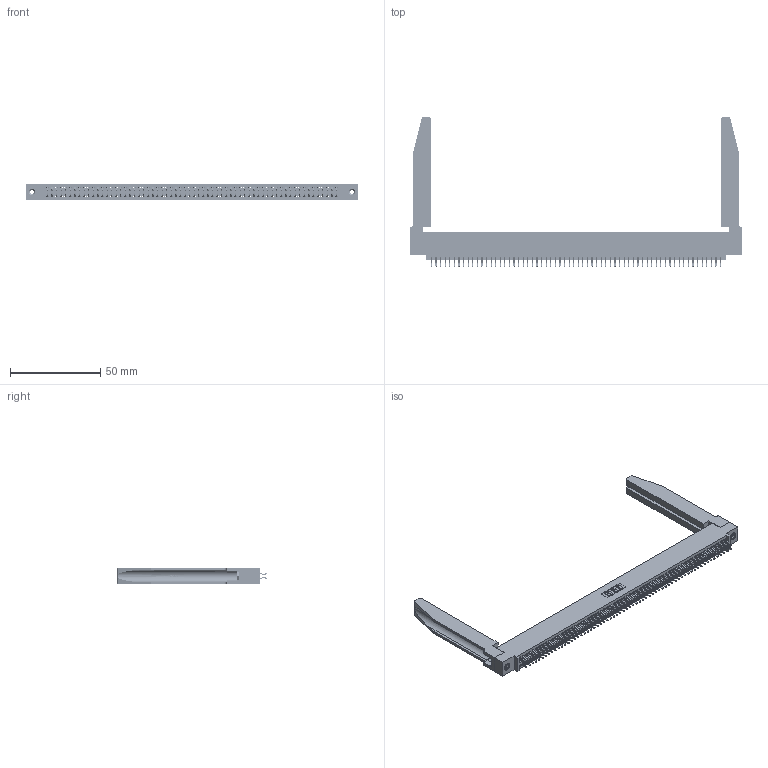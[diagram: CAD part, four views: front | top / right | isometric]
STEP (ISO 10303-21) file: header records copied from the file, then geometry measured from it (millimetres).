
FILE_DESCRIPTION (( 'STEP AP203' ), '1' );
FILE_NAME ('395-128-556-578.STEP', '2019-10-28T20:31:51', ( '' ), ( '' ), 'SwSTEP 2.0', 'SolidWorks 2016', '' );
FILE_SCHEMA (( 'CONFIG_CONTROL_DESIGN' ));
Length unit declared in the file: inch
Products named in the file (5): 345 Part_0.110 Offset - 0.156 Dia-TH; 345-292-001_556 Tail; 345-250-001_345-250-001-102; 345-220-078_345-220-078; 395-128-556-578
Assembly tree (133 placements, depth 2):
  395-128-556-578
    345 Part_0.110 Offset - 0.156 Dia-TH
    345-292-001_556 Tail  x128
    345-250-001_345-250-001-102  x2
    345-220-078_345-220-078  x2
Bounding box: 183.79 x 82.99 x 9.4 mm (x, y, z)
Volume: 25750.2 mm3; surface area: 33822.4 mm2
Topology: 133 solids, 133 shells, 7532 faces, 22337 edges, 14710 vertices
Faces by surface type: plane 4962, cylinder 2518, bspline 36, cone 12, torus 4
Entity records: 52346 total; most frequent: CARTESIAN_POINT 9687, ORIENTED_EDGE 8506, DIRECTION 7495, EDGE_CURVE 4253, LINE 3763, VECTOR 3763, VERTEX_POINT 2828, AXIS2_PLACEMENT_3D 1866
